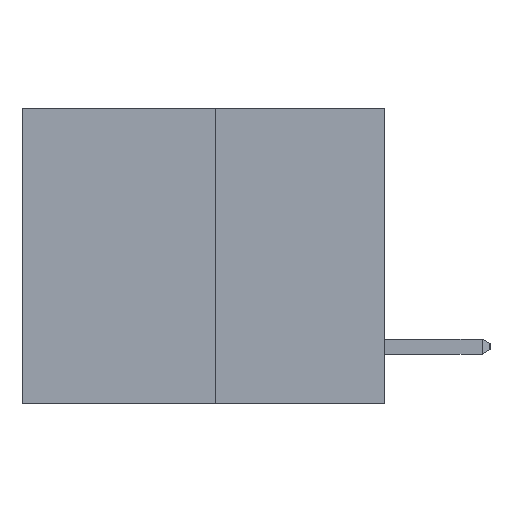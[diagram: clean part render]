
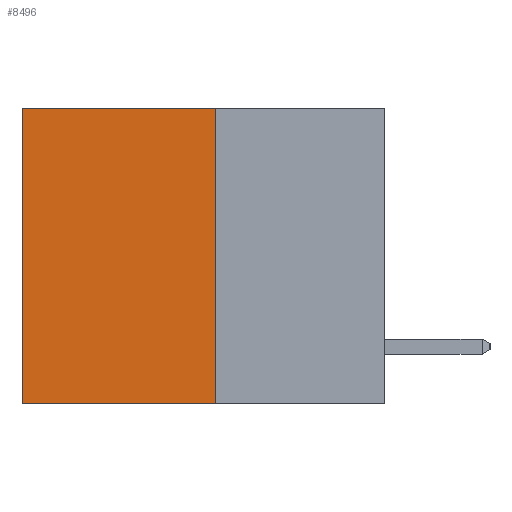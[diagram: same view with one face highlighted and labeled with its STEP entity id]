
A CAD part, left-side view. The second image highlights one B-rep face of the part: STEP entity #8496.
In plain terms, the highlighted planar face has unit normal (-1, 0, 0).
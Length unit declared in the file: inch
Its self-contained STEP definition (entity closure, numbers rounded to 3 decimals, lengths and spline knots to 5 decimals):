
#306 = VERTEX_POINT ( 'NONE', #1489 ) ;
#610 = EDGE_CURVE ( 'NONE', #11017, #2992, #6443, .T. ) ;
#879 = CARTESIAN_POINT ( 'NONE',  ( 0.3165, 0.6, -0.49 ) ) ;
#1489 = CARTESIAN_POINT ( 'NONE',  ( 0.3165, 0.6, 0. ) ) ;
#1802 = DIRECTION ( 'NONE',  ( 1., 0., 0. ) ) ;
#1878 = PLANE ( 'NONE',  #5862 ) ;
#2278 = DIRECTION ( 'NONE',  ( 0., 0., -1. ) ) ;
#2458 = ORIENTED_EDGE ( 'NONE', *, *, #9181, .T. ) ;
#2577 = ORIENTED_EDGE ( 'NONE', *, *, #10716, .F. ) ;
#2978 = DIRECTION ( 'NONE',  ( 0., 1., 0. ) ) ;
#2992 = VERTEX_POINT ( 'NONE', #9914 ) ;
#2993 = LINE ( 'NONE', #10159, #11879 ) ;
#3205 = CARTESIAN_POINT ( 'NONE',  ( 0.3165, 0.28, -0.49 ) ) ;
#3470 = VERTEX_POINT ( 'NONE', #879 ) ;
#3809 = VECTOR ( 'NONE', #11986, 39.37008 ) ;
#3942 = ORIENTED_EDGE ( 'NONE', *, *, #610, .F. ) ;
#5134 = VECTOR ( 'NONE', #2978, 39.37008 ) ;
#5304 = FACE_OUTER_BOUND ( 'NONE', #7911, .T. ) ;
#5609 = VECTOR ( 'NONE', #6333, 39.37008 ) ;
#5862 = AXIS2_PLACEMENT_3D ( 'NONE', #12547, #1802, #8686 ) ;
#6096 = CARTESIAN_POINT ( 'NONE',  ( 0.3165, 0.28, 0. ) ) ;
#6333 = DIRECTION ( 'NONE',  ( 0., 1., 0. ) ) ;
#6443 = LINE ( 'NONE', #3205, #3809 ) ;
#6588 = ORIENTED_EDGE ( 'NONE', *, *, #8895, .T. ) ;
#6808 = CARTESIAN_POINT ( 'NONE',  ( 0.3165, 0.28, 0. ) ) ;
#7777 = LINE ( 'NONE', #6808, #5134 ) ;
#7911 = EDGE_LOOP ( 'NONE', ( #2458, #2577, #3942, #6588 ) ) ;
#8251 = LINE ( 'NONE', #12151, #5609 ) ;
#8496 = ADVANCED_FACE ( 'NONE', ( #5304 ), #1878, .F. ) ;
#8686 = DIRECTION ( 'NONE',  ( 0., 0., -1. ) ) ;
#8895 = EDGE_CURVE ( 'NONE', #11017, #306, #7777, .T. ) ;
#9181 = EDGE_CURVE ( 'NONE', #306, #3470, #2993, .T. ) ;
#9914 = CARTESIAN_POINT ( 'NONE',  ( 0.3165, 0.28, -0.49 ) ) ;
#10159 = CARTESIAN_POINT ( 'NONE',  ( 0.3165, 0.6, -0.49 ) ) ;
#10716 = EDGE_CURVE ( 'NONE', #2992, #3470, #8251, .T. ) ;
#11017 = VERTEX_POINT ( 'NONE', #6096 ) ;
#11879 = VECTOR ( 'NONE', #2278, 39.37008 ) ;
#11986 = DIRECTION ( 'NONE',  ( 0., 0., -1. ) ) ;
#12151 = CARTESIAN_POINT ( 'NONE',  ( 0.3165, 0.28, -0.49 ) ) ;
#12547 = CARTESIAN_POINT ( 'NONE',  ( 0.3165, 0.28, -0.49 ) ) ;
